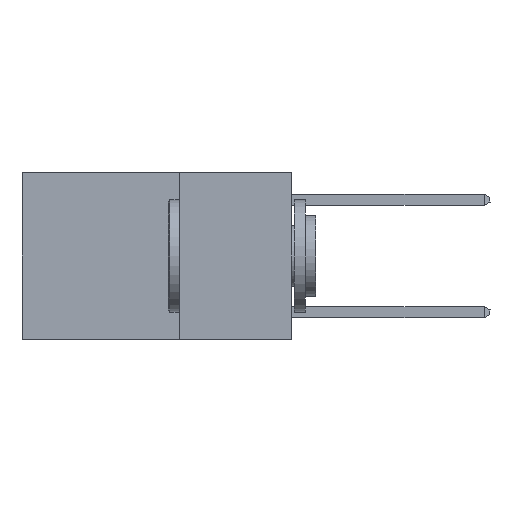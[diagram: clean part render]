
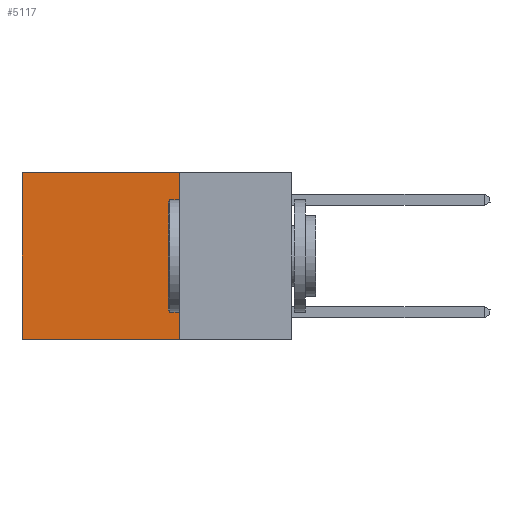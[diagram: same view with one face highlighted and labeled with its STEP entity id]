
A CAD part, left-side view. The second image highlights one B-rep face of the part: STEP entity #5117.
In plain terms, the highlighted planar face has unit normal (-1, 0, 0).
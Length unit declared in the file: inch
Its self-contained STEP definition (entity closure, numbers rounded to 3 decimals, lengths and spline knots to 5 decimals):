
#3733 = CARTESIAN_POINT ( 'NONE',  ( 0.2625, 0.25, 0. ) ) ;
#4195 = LINE ( 'NONE', #20207, #26771 ) ;
#4823 = EDGE_CURVE ( 'NONE', #11989, #10776, #4195, .T. ) ;
#4978 = EDGE_CURVE ( 'NONE', #10713, #10776, #8627, .T. ) ;
#5117 = ADVANCED_FACE ( 'NONE', ( #16263 ), #25075, .F. ) ;
#5265 = ORIENTED_EDGE ( 'NONE', *, *, #9996, .F. ) ;
#5819 = EDGE_LOOP ( 'NONE', ( #17819, #20271, #5265, #12457 ) ) ;
#6955 = DIRECTION ( 'NONE',  ( 0., 0., -1. ) ) ;
#7178 = VECTOR ( 'NONE', #13261, 39.37008 ) ;
#8627 = LINE ( 'NONE', #15652, #7178 ) ;
#8638 = VERTEX_POINT ( 'NONE', #27460 ) ;
#8852 = CARTESIAN_POINT ( 'NONE',  ( 0.2625, 0.6, 0. ) ) ;
#8981 = DIRECTION ( 'NONE',  ( 0., 0., -1. ) ) ;
#8990 = EDGE_CURVE ( 'NONE', #8638, #11989, #24014, .T. ) ;
#9996 = EDGE_CURVE ( 'NONE', #8638, #10713, #18728, .T. ) ;
#10165 = DIRECTION ( 'NONE',  ( 0., 0., -1. ) ) ;
#10713 = VERTEX_POINT ( 'NONE', #29007 ) ;
#10776 = VERTEX_POINT ( 'NONE', #16315 ) ;
#11596 = CARTESIAN_POINT ( 'NONE',  ( 0.2625, 0.25, 0. ) ) ;
#11989 = VERTEX_POINT ( 'NONE', #8852 ) ;
#12457 = ORIENTED_EDGE ( 'NONE', *, *, #8990, .T. ) ;
#13261 = DIRECTION ( 'NONE',  ( 0., 1., 0. ) ) ;
#15652 = CARTESIAN_POINT ( 'NONE',  ( 0.2625, 0.25, -0.37 ) ) ;
#15816 = AXIS2_PLACEMENT_3D ( 'NONE', #11596, #25378, #6955 ) ;
#16263 = FACE_OUTER_BOUND ( 'NONE', #5819, .T. ) ;
#16315 = CARTESIAN_POINT ( 'NONE',  ( 0.2625, 0.6, -0.37 ) ) ;
#17819 = ORIENTED_EDGE ( 'NONE', *, *, #4823, .T. ) ;
#18111 = VECTOR ( 'NONE', #21777, 39.37008 ) ;
#18728 = LINE ( 'NONE', #3733, #28165 ) ;
#19823 = CARTESIAN_POINT ( 'NONE',  ( 0.2625, 0.25, 0. ) ) ;
#20207 = CARTESIAN_POINT ( 'NONE',  ( 0.2625, 0.6, 0. ) ) ;
#20271 = ORIENTED_EDGE ( 'NONE', *, *, #4978, .F. ) ;
#21777 = DIRECTION ( 'NONE',  ( 0., 1., 0. ) ) ;
#24014 = LINE ( 'NONE', #19823, #18111 ) ;
#25075 = PLANE ( 'NONE',  #15816 ) ;
#25378 = DIRECTION ( 'NONE',  ( 1., 0., 0. ) ) ;
#26771 = VECTOR ( 'NONE', #8981, 39.37008 ) ;
#27460 = CARTESIAN_POINT ( 'NONE',  ( 0.2625, 0.25, 0. ) ) ;
#28165 = VECTOR ( 'NONE', #10165, 39.37008 ) ;
#29007 = CARTESIAN_POINT ( 'NONE',  ( 0.2625, 0.25, -0.37 ) ) ;
